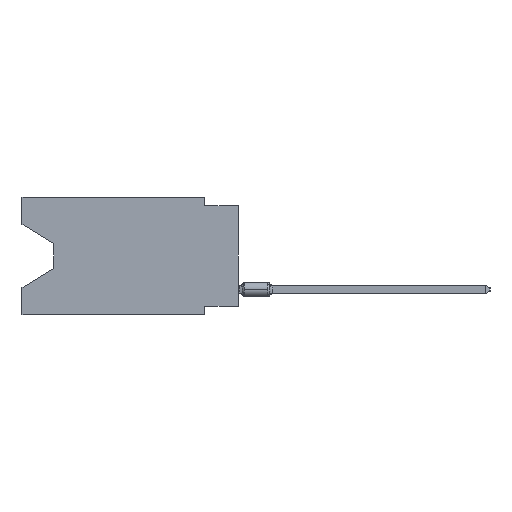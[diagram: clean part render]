
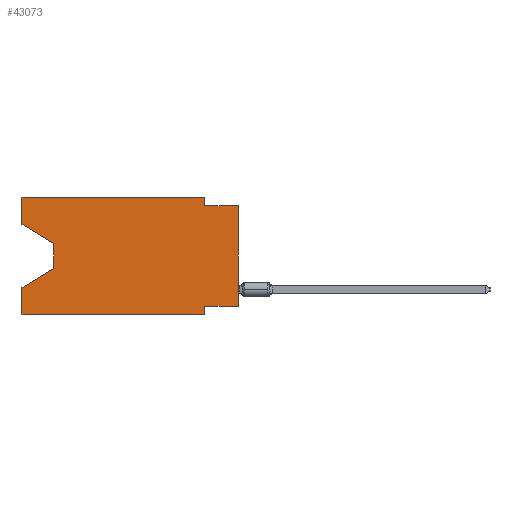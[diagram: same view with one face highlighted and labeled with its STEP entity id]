
A CAD part, left-side view. The second image highlights one B-rep face of the part: STEP entity #43073.
In plain terms, the highlighted planar face has unit normal (-1, 0, 0).
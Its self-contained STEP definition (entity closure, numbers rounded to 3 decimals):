
#434 = CARTESIAN_POINT ( 'NONE',  ( 0., 0., -0.635 ) ) ;
#469 = ORIENTED_EDGE ( 'NONE', *, *, #22968, .F. ) ;
#1630 = VERTEX_POINT ( 'NONE', #10790 ) ;
#3714 = VECTOR ( 'NONE', #37262, 1000. ) ;
#3790 = EDGE_CURVE ( 'NONE', #44977, #22619, #44251, .T. ) ;
#3829 = VERTEX_POINT ( 'NONE', #37521 ) ;
#3975 = CARTESIAN_POINT ( 'NONE',  ( 0., 2.54, -8.255 ) ) ;
#4179 = LINE ( 'NONE', #11833, #31071 ) ;
#4502 = CARTESIAN_POINT ( 'NONE',  ( 0., 2.54, -8.89 ) ) ;
#4606 = PLANE ( 'NONE',  #20476 ) ;
#4832 = FACE_OUTER_BOUND ( 'NONE', #34068, .T. ) ;
#6245 = CARTESIAN_POINT ( 'NONE',  ( 0., 2.54, -8.89 ) ) ;
#7646 = DIRECTION ( 'NONE',  ( 0., -0.855, -0.519 ) ) ;
#7793 = CARTESIAN_POINT ( 'NONE',  ( 0., 13.97, -5.385 ) ) ;
#7911 = DIRECTION ( 'NONE',  ( 0., -1., 0. ) ) ;
#7936 = VERTEX_POINT ( 'NONE', #28764 ) ;
#8200 = VECTOR ( 'NONE', #12601, 1000. ) ;
#9338 = CARTESIAN_POINT ( 'NONE',  ( 0., 0., -8.255 ) ) ;
#10790 = CARTESIAN_POINT ( 'NONE',  ( 0., 16.383, 0. ) ) ;
#11621 = VERTEX_POINT ( 'NONE', #24063 ) ;
#11833 = CARTESIAN_POINT ( 'NONE',  ( 0., 16.383, -2.038 ) ) ;
#12601 = DIRECTION ( 'NONE',  ( 0., 0., -1. ) ) ;
#12714 = EDGE_CURVE ( 'NONE', #26117, #11621, #4179, .T. ) ;
#13073 = LINE ( 'NONE', #9338, #3714 ) ;
#13182 = DIRECTION ( 'NONE',  ( 0., -1., 0. ) ) ;
#13463 = LINE ( 'NONE', #26947, #36065 ) ;
#14989 = ORIENTED_EDGE ( 'NONE', *, *, #34004, .T. ) ;
#15020 = LINE ( 'NONE', #7793, #27899 ) ;
#15023 = CARTESIAN_POINT ( 'NONE',  ( 0., 2.54, 0. ) ) ;
#15131 = CARTESIAN_POINT ( 'NONE',  ( 0., 16.383, -2.038 ) ) ;
#15630 = VECTOR ( 'NONE', #7911, 1000. ) ;
#16058 = ORIENTED_EDGE ( 'NONE', *, *, #42964, .T. ) ;
#16157 = VECTOR ( 'NONE', #41545, 1000. ) ;
#16372 = CARTESIAN_POINT ( 'NONE',  ( 0., 16.383, 0. ) ) ;
#16496 = CARTESIAN_POINT ( 'NONE',  ( 0., 2.54, 0. ) ) ;
#16497 = DIRECTION ( 'NONE',  ( 0., -1., 0. ) ) ;
#17187 = DIRECTION ( 'NONE',  ( 0., 0., -1. ) ) ;
#18083 = VERTEX_POINT ( 'NONE', #4502 ) ;
#18312 = ORIENTED_EDGE ( 'NONE', *, *, #28037, .F. ) ;
#18782 = ORIENTED_EDGE ( 'NONE', *, *, #41198, .F. ) ;
#19039 = DIRECTION ( 'NONE',  ( 1., 0., 0. ) ) ;
#19426 = ORIENTED_EDGE ( 'NONE', *, *, #3790, .F. ) ;
#20476 = AXIS2_PLACEMENT_3D ( 'NONE', #28808, #19039, #25085 ) ;
#20964 = CARTESIAN_POINT ( 'NONE',  ( 0., 0., 0. ) ) ;
#21371 = VERTEX_POINT ( 'NONE', #3975 ) ;
#22619 = VERTEX_POINT ( 'NONE', #24152 ) ;
#22968 = EDGE_CURVE ( 'NONE', #27275, #43143, #30852, .T. ) ;
#24063 = CARTESIAN_POINT ( 'NONE',  ( 0., 13.97, -3.505 ) ) ;
#24152 = CARTESIAN_POINT ( 'NONE',  ( 0., 16.383, -6.852 ) ) ;
#24423 = EDGE_CURVE ( 'NONE', #3829, #22619, #15020, .T. ) ;
#25085 = DIRECTION ( 'NONE',  ( 0., 0., -1. ) ) ;
#25902 = CARTESIAN_POINT ( 'NONE',  ( 0., 16.383, -8.89 ) ) ;
#25914 = DIRECTION ( 'NONE',  ( 0., 0.855, -0.519 ) ) ;
#26030 = EDGE_CURVE ( 'NONE', #26117, #1630, #27347, .T. ) ;
#26117 = VERTEX_POINT ( 'NONE', #15131 ) ;
#26947 = CARTESIAN_POINT ( 'NONE',  ( 0., 16.383, -8.89 ) ) ;
#27051 = DIRECTION ( 'NONE',  ( 0., 0., 1. ) ) ;
#27275 = VERTEX_POINT ( 'NONE', #40612 ) ;
#27347 = LINE ( 'NONE', #44786, #16157 ) ;
#27899 = VECTOR ( 'NONE', #25914, 1000. ) ;
#28037 = EDGE_CURVE ( 'NONE', #21371, #18083, #43973, .T. ) ;
#28625 = ORIENTED_EDGE ( 'NONE', *, *, #30982, .F. ) ;
#28764 = CARTESIAN_POINT ( 'NONE',  ( 0., 0., -8.255 ) ) ;
#28808 = CARTESIAN_POINT ( 'NONE',  ( 0., 16.383, 0. ) ) ;
#29079 = CARTESIAN_POINT ( 'NONE',  ( 0., 16.383, 0. ) ) ;
#30852 = LINE ( 'NONE', #45014, #36011 ) ;
#30910 = LINE ( 'NONE', #16496, #32232 ) ;
#30982 = EDGE_CURVE ( 'NONE', #41794, #27275, #30910, .T. ) ;
#31071 = VECTOR ( 'NONE', #7646, 1000. ) ;
#31169 = CARTESIAN_POINT ( 'NONE',  ( 0., 13.97, -3.505 ) ) ;
#31657 = LINE ( 'NONE', #20964, #32334 ) ;
#32232 = VECTOR ( 'NONE', #17187, 1000. ) ;
#32334 = VECTOR ( 'NONE', #45798, 1000. ) ;
#32587 = LINE ( 'NONE', #29079, #15630 ) ;
#34004 = EDGE_CURVE ( 'NONE', #7936, #43143, #31657, .T. ) ;
#34068 = EDGE_LOOP ( 'NONE', ( #36723, #16058, #37819, #19426, #40325, #18312, #18782, #14989, #469, #28625, #40771, #36949 ) ) ;
#36011 = VECTOR ( 'NONE', #13182, 1000. ) ;
#36065 = VECTOR ( 'NONE', #16497, 1000. ) ;
#36723 = ORIENTED_EDGE ( 'NONE', *, *, #12714, .T. ) ;
#36949 = ORIENTED_EDGE ( 'NONE', *, *, #26030, .F. ) ;
#37262 = DIRECTION ( 'NONE',  ( 0., 1., 0. ) ) ;
#37521 = CARTESIAN_POINT ( 'NONE',  ( 0., 13.97, -5.385 ) ) ;
#37819 = ORIENTED_EDGE ( 'NONE', *, *, #24423, .T. ) ;
#38127 = LINE ( 'NONE', #31169, #38271 ) ;
#38271 = VECTOR ( 'NONE', #38589, 1000. ) ;
#38589 = DIRECTION ( 'NONE',  ( 0., 0., -1. ) ) ;
#40325 = ORIENTED_EDGE ( 'NONE', *, *, #44196, .T. ) ;
#40612 = CARTESIAN_POINT ( 'NONE',  ( 0., 2.54, -0.635 ) ) ;
#40771 = ORIENTED_EDGE ( 'NONE', *, *, #41479, .F. ) ;
#41198 = EDGE_CURVE ( 'NONE', #7936, #21371, #13073, .T. ) ;
#41479 = EDGE_CURVE ( 'NONE', #1630, #41794, #32587, .T. ) ;
#41545 = DIRECTION ( 'NONE',  ( 0., 0., 1. ) ) ;
#41794 = VERTEX_POINT ( 'NONE', #15023 ) ;
#42366 = VECTOR ( 'NONE', #27051, 1000. ) ;
#42964 = EDGE_CURVE ( 'NONE', #11621, #3829, #38127, .T. ) ;
#43073 = ADVANCED_FACE ( 'NONE', ( #4832 ), #4606, .F. ) ;
#43143 = VERTEX_POINT ( 'NONE', #434 ) ;
#43973 = LINE ( 'NONE', #6245, #8200 ) ;
#44196 = EDGE_CURVE ( 'NONE', #44977, #18083, #13463, .T. ) ;
#44251 = LINE ( 'NONE', #16372, #42366 ) ;
#44786 = CARTESIAN_POINT ( 'NONE',  ( 0., 16.383, 0. ) ) ;
#44977 = VERTEX_POINT ( 'NONE', #25902 ) ;
#45014 = CARTESIAN_POINT ( 'NONE',  ( 0., 0., -0.635 ) ) ;
#45798 = DIRECTION ( 'NONE',  ( 0., 0., 1. ) ) ;
